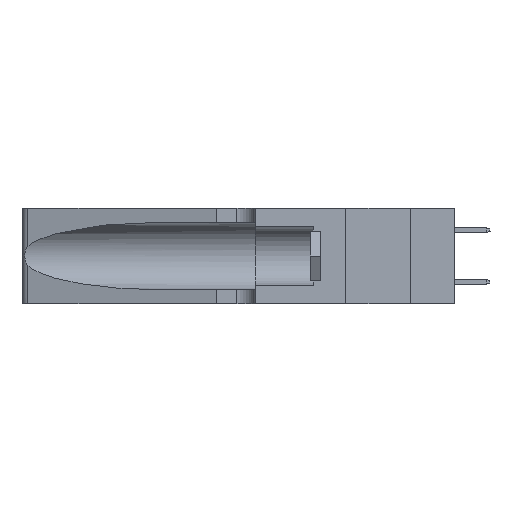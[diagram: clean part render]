
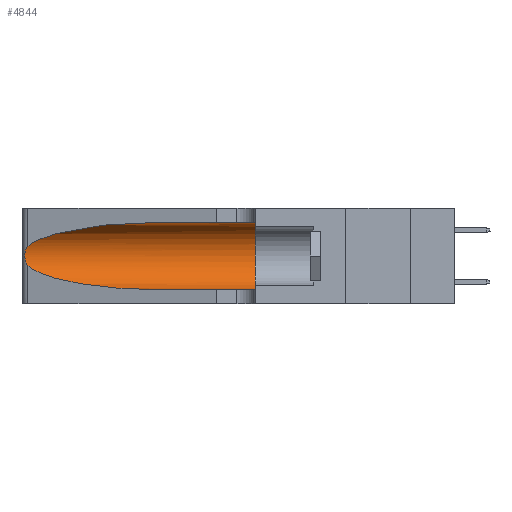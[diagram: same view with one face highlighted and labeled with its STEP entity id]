
A CAD part, left-side view. The second image highlights one B-rep face of the part: STEP entity #4844.
In plain terms, the highlighted cylindrical face has radius 3.308 mm (diameter 6.617 mm), a partial arc.
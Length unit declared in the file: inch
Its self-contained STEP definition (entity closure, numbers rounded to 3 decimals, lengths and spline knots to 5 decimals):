
#1187 = CARTESIAN_POINT ( 'NONE',  ( 0.25487, 1.22718, 0.14631 ) ) ;
#1198 = VERTEX_POINT ( 'NONE', #5514 ) ;
#1561 = CARTESIAN_POINT ( 'NONE',  ( 0.18966, 0.96281, 0.31525 ) ) ;
#1631 = VERTEX_POINT ( 'NONE', #11996 ) ;
#2346 = AXIS2_PLACEMENT_3D ( 'NONE', #8774, #3759, #16439 ) ;
#3123 = CARTESIAN_POINT ( 'NONE',  ( 0.26017, 1.23833, 0.17102 ) ) ;
#3759 = DIRECTION ( 'NONE',  ( 0., -1., 0. ) ) ;
#3863 = CARTESIAN_POINT ( 'NONE',  ( 0.1305, 1.61858, 0.05475 ) ) ;
#4614 = DIRECTION ( 'NONE',  ( 0., 0., 1. ) ) ;
#4844 = ADVANCED_FACE ( 'NONE', ( #28136 ), #18375, .F. ) ;
#5514 = CARTESIAN_POINT ( 'NONE',  ( 0.25487, 1.22718, 0.22369 ) ) ;
#5555 = CARTESIAN_POINT ( 'NONE',  ( 0.25639, 1.23186, 0.15144 ) ) ;
#5757 = DIRECTION ( 'NONE',  ( 0., -1., 0. ) ) ;
#7935 = CARTESIAN_POINT ( 'NONE',  ( 0.1305, 0.35, 0.31525 ) ) ;
#8107 = VERTEX_POINT ( 'NONE', #17355 ) ;
#8774 = CARTESIAN_POINT ( 'NONE',  ( 0.1305, 1.61858, 0.185 ) ) ;
#8823 = EDGE_CURVE ( 'NONE', #8107, #9493, #23320, .T. ) ;
#9342 = ORIENTED_EDGE ( 'NONE', *, *, #31018, .T. ) ;
#9351 = CIRCLE ( 'NONE', #16146, 0.13025 ) ;
#9493 = VERTEX_POINT ( 'NONE', #7935 ) ;
#10078 =( BOUNDED_CURVE ( )  B_SPLINE_CURVE ( 3, ( #21099, #1561, #15876, #21433 ),
 .UNSPECIFIED., .F., .T. ) 
 B_SPLINE_CURVE_WITH_KNOTS ( ( 4, 4 ),
 ( 1.5708, 2.84003 ),
 .UNSPECIFIED. ) 
 CURVE ( )  GEOMETRIC_REPRESENTATION_ITEM ( )  RATIONAL_B_SPLINE_CURVE ( ( 1., 0.87, 0.87, 1. ) ) 
 REPRESENTATION_ITEM ( '' )  );
#10275 = CARTESIAN_POINT ( 'NONE',  ( 0.26075, 1.23896, 0.19203 ) ) ;
#10607 = CARTESIAN_POINT ( 'NONE',  ( 0.25487, 1.22718, 0.22369 ) ) ;
#10754 = CARTESIAN_POINT ( 'NONE',  ( 0.25789, 1.23486, 0.15765 ) ) ;
#11413 = CARTESIAN_POINT ( 'NONE',  ( 0.1305, 0.72297, 0.05475 ) ) ;
#11923 = DIRECTION ( 'NONE',  ( 0., 1., 0. ) ) ;
#11996 = CARTESIAN_POINT ( 'NONE',  ( 0.1305, 0.72297, 0.05475 ) ) ;
#12544 = CARTESIAN_POINT ( 'NONE',  ( 0.25639, 1.23184, 0.21858 ) ) ;
#12861 = EDGE_CURVE ( 'NONE', #8107, #1198, #10078, .T. ) ;
#13044 = CARTESIAN_POINT ( 'NONE',  ( 0.25487, 1.22718, 0.14631 ) ) ;
#13166 = VECTOR ( 'NONE', #23858, 39.37008 ) ;
#13207 = CARTESIAN_POINT ( 'NONE',  ( 0.25856, 1.23593, 0.16098 ) ) ;
#13973 = VECTOR ( 'NONE', #5757, 39.37008 ) ;
#14228 = EDGE_LOOP ( 'NONE', ( #28737, #30254, #16462, #9342, #24570, #23058 ) ) ;
#15829 = CARTESIAN_POINT ( 'NONE',  ( 0.18966, 0.96281, 0.05475 ) ) ;
#15876 = CARTESIAN_POINT ( 'NONE',  ( 0.2373, 1.15595, 0.28018 ) ) ;
#16146 = AXIS2_PLACEMENT_3D ( 'NONE', #22046, #11923, #4614 ) ;
#16439 = DIRECTION ( 'NONE',  ( 0., 0., -1. ) ) ;
#16462 = ORIENTED_EDGE ( 'NONE', *, *, #20874, .T. ) ;
#16550 = LINE ( 'NONE', #3863, #13166 ) ;
#17355 = CARTESIAN_POINT ( 'NONE',  ( 0.1305, 0.72297, 0.31525 ) ) ;
#17421 = CARTESIAN_POINT ( 'NONE',  ( 0.1305, 0.35, 0.05475 ) ) ;
#17437 = CARTESIAN_POINT ( 'NONE',  ( 0.26018, 1.23835, 0.19895 ) ) ;
#17911 = CARTESIAN_POINT ( 'NONE',  ( 0.26075, 1.23896, 0.178 ) ) ;
#18375 = CYLINDRICAL_SURFACE ( 'NONE', #2346, 0.13025 ) ;
#18399 = CARTESIAN_POINT ( 'NONE',  ( 0.2373, 1.15595, 0.08982 ) ) ;
#18814 = CARTESIAN_POINT ( 'NONE',  ( 0.25487, 1.22718, 0.14631 ) ) ;
#19895 =( BOUNDED_CURVE ( )  B_SPLINE_CURVE ( 3, ( #1187, #18399, #15829, #11413 ),
 .UNSPECIFIED., .F., .T. ) 
 B_SPLINE_CURVE_WITH_KNOTS ( ( 4, 4 ),
 ( 3.44316, 4.71239 ),
 .UNSPECIFIED. ) 
 CURVE ( )  GEOMETRIC_REPRESENTATION_ITEM ( )  RATIONAL_B_SPLINE_CURVE ( ( 1., 0.87, 0.87, 1. ) ) 
 REPRESENTATION_ITEM ( '' )  );
#20222 = CARTESIAN_POINT ( 'NONE',  ( 0.25555, 1.22993, 0.14849 ) ) ;
#20725 = EDGE_CURVE ( 'NONE', #1198, #25138, #21135, .T. ) ;
#20874 = EDGE_CURVE ( 'NONE', #25138, #1631, #19895, .T. ) ;
#21099 = CARTESIAN_POINT ( 'NONE',  ( 0.1305, 0.72297, 0.31525 ) ) ;
#21135 = B_SPLINE_CURVE_WITH_KNOTS ( 'NONE', 3,
 ( #10607, #22507, #12544, #22980, #30106, #17437, #10275, #17911, #3123, #13207, #10754, #5555, #20222, #13044 ),
 .UNSPECIFIED., .F., .F.,
 ( 4, 2, 2, 2, 2, 2, 4 ),
 ( 0., 0.00027, 0.00053, 0.00107, 0.0016, 0.00187, 0.00214 ),
 .UNSPECIFIED. ) ;
#21433 = CARTESIAN_POINT ( 'NONE',  ( 0.25487, 1.22718, 0.22369 ) ) ;
#22046 = CARTESIAN_POINT ( 'NONE',  ( 0.1305, 0.35, 0.185 ) ) ;
#22494 = VERTEX_POINT ( 'NONE', #17421 ) ;
#22507 = CARTESIAN_POINT ( 'NONE',  ( 0.25555, 1.22994, 0.2215 ) ) ;
#22980 = CARTESIAN_POINT ( 'NONE',  ( 0.25787, 1.23484, 0.2124 ) ) ;
#23058 = ORIENTED_EDGE ( 'NONE', *, *, #8823, .F. ) ;
#23320 = LINE ( 'NONE', #28510, #13973 ) ;
#23858 = DIRECTION ( 'NONE',  ( 0., -1., 0. ) ) ;
#24570 = ORIENTED_EDGE ( 'NONE', *, *, #27223, .F. ) ;
#25138 = VERTEX_POINT ( 'NONE', #18814 ) ;
#27223 = EDGE_CURVE ( 'NONE', #9493, #22494, #9351, .T. ) ;
#28136 = FACE_OUTER_BOUND ( 'NONE', #14228, .T. ) ;
#28510 = CARTESIAN_POINT ( 'NONE',  ( 0.1305, 1.61858, 0.31525 ) ) ;
#28737 = ORIENTED_EDGE ( 'NONE', *, *, #12861, .T. ) ;
#30106 = CARTESIAN_POINT ( 'NONE',  ( 0.25854, 1.2359, 0.20912 ) ) ;
#30254 = ORIENTED_EDGE ( 'NONE', *, *, #20725, .T. ) ;
#31018 = EDGE_CURVE ( 'NONE', #1631, #22494, #16550, .T. ) ;
